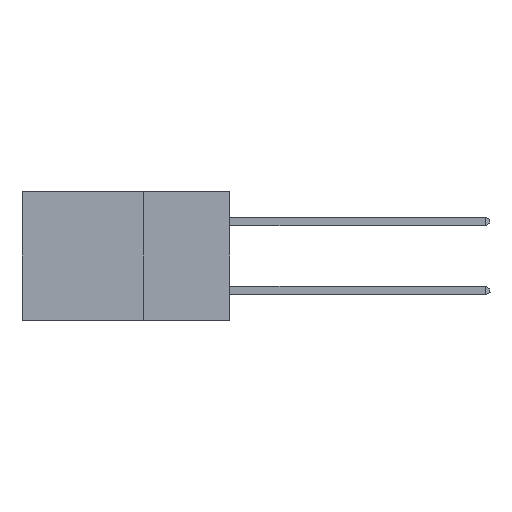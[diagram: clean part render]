
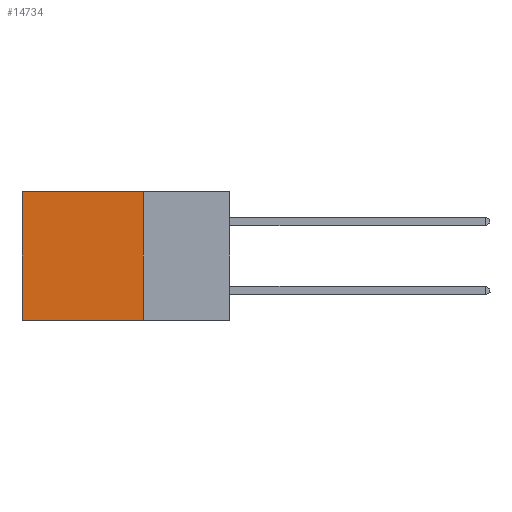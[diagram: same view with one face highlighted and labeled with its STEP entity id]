
A CAD part, left-side view. The second image highlights one B-rep face of the part: STEP entity #14734.
In plain terms, the highlighted planar face has unit normal (-1, 0, 0).
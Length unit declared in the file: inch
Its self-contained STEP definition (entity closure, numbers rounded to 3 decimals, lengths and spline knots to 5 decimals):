
#296 = DIRECTION ( 'NONE',  ( 1., 0., 0. ) ) ;
#2492 = EDGE_CURVE ( 'NONE', #24628, #12148, #7595, .T. ) ;
#2781 = ORIENTED_EDGE ( 'NONE', *, *, #19490, .T. ) ;
#4506 = DIRECTION ( 'NONE',  ( 0., 1., 0. ) ) ;
#4877 = FACE_OUTER_BOUND ( 'NONE', #22139, .T. ) ;
#5859 = LINE ( 'NONE', #16454, #15173 ) ;
#7589 = CARTESIAN_POINT ( 'NONE',  ( 0.298, 0.25, 0. ) ) ;
#7595 = LINE ( 'NONE', #7589, #22176 ) ;
#7809 = CARTESIAN_POINT ( 'NONE',  ( 0.298, 0.25, -0.37 ) ) ;
#8249 = CARTESIAN_POINT ( 'NONE',  ( 0.298, 0.25, -0.37 ) ) ;
#8635 = VECTOR ( 'NONE', #4506, 39.37008 ) ;
#9934 = CARTESIAN_POINT ( 'NONE',  ( 0.298, 0.25, 0. ) ) ;
#10187 = PLANE ( 'NONE',  #18065 ) ;
#10810 = CARTESIAN_POINT ( 'NONE',  ( 0.298, 0.6, -0.37 ) ) ;
#10949 = EDGE_CURVE ( 'NONE', #24628, #16644, #5859, .T. ) ;
#11230 = CARTESIAN_POINT ( 'NONE',  ( 0.298, 0.6, 0. ) ) ;
#11759 = LINE ( 'NONE', #8249, #8635 ) ;
#12148 = VERTEX_POINT ( 'NONE', #7809 ) ;
#13073 = VERTEX_POINT ( 'NONE', #10810 ) ;
#13989 = DIRECTION ( 'NONE',  ( 0., 0., -1. ) ) ;
#14734 = ADVANCED_FACE ( 'NONE', ( #4877 ), #10187, .F. ) ;
#15173 = VECTOR ( 'NONE', #18275, 39.37008 ) ;
#15185 = CARTESIAN_POINT ( 'NONE',  ( 0.298, 0.25, 0. ) ) ;
#15516 = DIRECTION ( 'NONE',  ( 0., 0., -1. ) ) ;
#16454 = CARTESIAN_POINT ( 'NONE',  ( 0.298, 0.25, 0. ) ) ;
#16644 = VERTEX_POINT ( 'NONE', #11230 ) ;
#18026 = LINE ( 'NONE', #22484, #20387 ) ;
#18065 = AXIS2_PLACEMENT_3D ( 'NONE', #9934, #296, #13989 ) ;
#18275 = DIRECTION ( 'NONE',  ( 0., 1., 0. ) ) ;
#19490 = EDGE_CURVE ( 'NONE', #16644, #13073, #18026, .T. ) ;
#19999 = EDGE_CURVE ( 'NONE', #12148, #13073, #11759, .T. ) ;
#20387 = VECTOR ( 'NONE', #21950, 39.37008 ) ;
#20792 = ORIENTED_EDGE ( 'NONE', *, *, #10949, .T. ) ;
#21682 = ORIENTED_EDGE ( 'NONE', *, *, #19999, .F. ) ;
#21837 = ORIENTED_EDGE ( 'NONE', *, *, #2492, .F. ) ;
#21950 = DIRECTION ( 'NONE',  ( 0., 0., -1. ) ) ;
#22139 = EDGE_LOOP ( 'NONE', ( #2781, #21682, #21837, #20792 ) ) ;
#22176 = VECTOR ( 'NONE', #15516, 39.37008 ) ;
#22484 = CARTESIAN_POINT ( 'NONE',  ( 0.298, 0.6, 0. ) ) ;
#24628 = VERTEX_POINT ( 'NONE', #15185 ) ;
